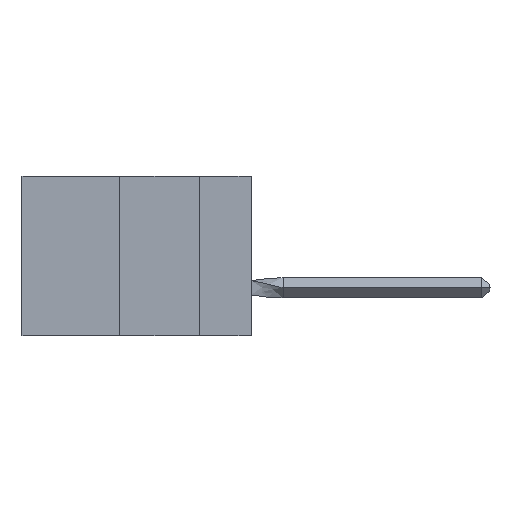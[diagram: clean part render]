
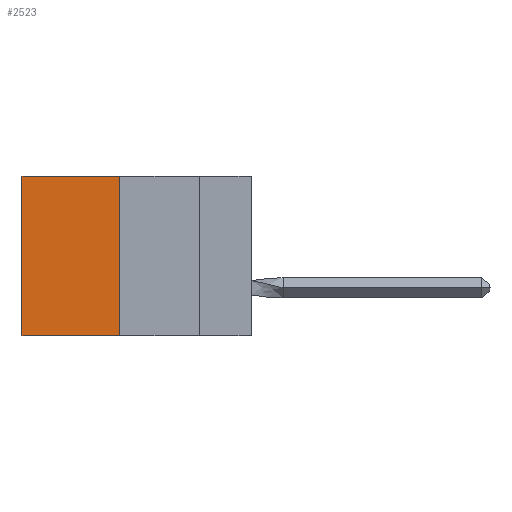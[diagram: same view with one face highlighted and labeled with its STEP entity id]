
A CAD part, left-side view. The second image highlights one B-rep face of the part: STEP entity #2523.
In plain terms, the highlighted planar face has unit normal (-1, 0, 0).
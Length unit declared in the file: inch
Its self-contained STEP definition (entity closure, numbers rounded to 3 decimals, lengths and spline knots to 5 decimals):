
#1502 = CARTESIAN_POINT ( 'NONE',  ( 0.305, 0.72, -0.5 ) ) ;
#2056 = CARTESIAN_POINT ( 'NONE',  ( 0.305, 0.413, 0. ) ) ;
#2133 = DIRECTION ( 'NONE',  ( 1., 0., 0. ) ) ;
#2523 = ADVANCED_FACE ( 'NONE', ( #13619 ), #18245, .F. ) ;
#2741 = CARTESIAN_POINT ( 'NONE',  ( 0.305, 0.72, -0.5 ) ) ;
#3050 = EDGE_CURVE ( 'NONE', #6877, #12057, #14710, .T. ) ;
#3601 = ORIENTED_EDGE ( 'NONE', *, *, #4893, .T. ) ;
#4825 = CARTESIAN_POINT ( 'NONE',  ( 0.305, 0.72, 0. ) ) ;
#4893 = EDGE_CURVE ( 'NONE', #7753, #12057, #13086, .T. ) ;
#5619 = VECTOR ( 'NONE', #10605, 39.37008 ) ;
#5832 = VERTEX_POINT ( 'NONE', #9822 ) ;
#6877 = VERTEX_POINT ( 'NONE', #14939 ) ;
#7193 = EDGE_CURVE ( 'NONE', #5832, #7753, #15782, .T. ) ;
#7753 = VERTEX_POINT ( 'NONE', #4825 ) ;
#7864 = ORIENTED_EDGE ( 'NONE', *, *, #7193, .T. ) ;
#8863 = DIRECTION ( 'NONE',  ( 0., 0., -1. ) ) ;
#9550 = CARTESIAN_POINT ( 'NONE',  ( 0.305, 0.413, -0.5 ) ) ;
#9608 = DIRECTION ( 'NONE',  ( 0., 0., -1. ) ) ;
#9822 = CARTESIAN_POINT ( 'NONE',  ( 0.305, 0.413, 0. ) ) ;
#10605 = DIRECTION ( 'NONE',  ( 0., 1., 0. ) ) ;
#10877 = AXIS2_PLACEMENT_3D ( 'NONE', #9550, #2133, #9608 ) ;
#10884 = VECTOR ( 'NONE', #18110, 39.37008 ) ;
#12057 = VERTEX_POINT ( 'NONE', #2741 ) ;
#12365 = CARTESIAN_POINT ( 'NONE',  ( 0.305, 0.413, -0.5 ) ) ;
#12714 = CARTESIAN_POINT ( 'NONE',  ( 0.305, 0.413, -0.5 ) ) ;
#13086 = LINE ( 'NONE', #1502, #13309 ) ;
#13309 = VECTOR ( 'NONE', #8863, 39.37008 ) ;
#13461 = EDGE_LOOP ( 'NONE', ( #3601, #17834, #14919, #7864 ) ) ;
#13619 = FACE_OUTER_BOUND ( 'NONE', #13461, .T. ) ;
#14388 = VECTOR ( 'NONE', #16984, 39.37008 ) ;
#14710 = LINE ( 'NONE', #12365, #10884 ) ;
#14919 = ORIENTED_EDGE ( 'NONE', *, *, #18463, .F. ) ;
#14939 = CARTESIAN_POINT ( 'NONE',  ( 0.305, 0.413, -0.5 ) ) ;
#15782 = LINE ( 'NONE', #2056, #5619 ) ;
#16181 = LINE ( 'NONE', #12714, #14388 ) ;
#16984 = DIRECTION ( 'NONE',  ( 0., 0., -1. ) ) ;
#17834 = ORIENTED_EDGE ( 'NONE', *, *, #3050, .F. ) ;
#18110 = DIRECTION ( 'NONE',  ( 0., 1., 0. ) ) ;
#18245 = PLANE ( 'NONE',  #10877 ) ;
#18463 = EDGE_CURVE ( 'NONE', #5832, #6877, #16181, .T. ) ;
